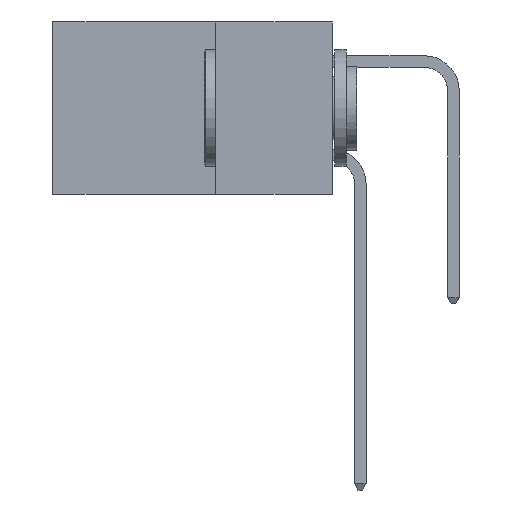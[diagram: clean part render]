
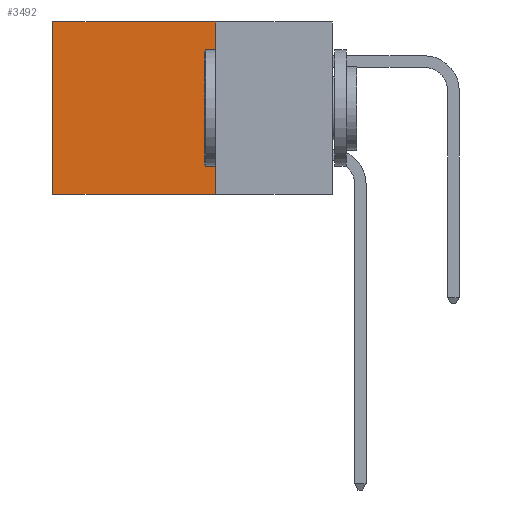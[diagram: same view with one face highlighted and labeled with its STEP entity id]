
A CAD part, left-side view. The second image highlights one B-rep face of the part: STEP entity #3492.
In plain terms, the highlighted planar face has unit normal (-1, 0, 0).
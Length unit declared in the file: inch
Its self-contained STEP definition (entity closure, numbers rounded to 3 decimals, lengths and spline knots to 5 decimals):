
#49 = CARTESIAN_POINT ( 'NONE',  ( 0.2615, 0.6, -0.37 ) ) ;
#805 = LINE ( 'NONE', #8784, #5209 ) ;
#1521 = EDGE_CURVE ( 'NONE', #4899, #5597, #2468, .T. ) ;
#1525 = CARTESIAN_POINT ( 'NONE',  ( 0.2615, 0.25, -0.37 ) ) ;
#1537 = DIRECTION ( 'NONE',  ( 0., 0., -1. ) ) ;
#1586 = DIRECTION ( 'NONE',  ( 1., 0., 0. ) ) ;
#1589 = PLANE ( 'NONE',  #4593 ) ;
#1717 = DIRECTION ( 'NONE',  ( 0., 1., 0. ) ) ;
#1936 = CARTESIAN_POINT ( 'NONE',  ( 0.2615, 0.25, -0.37 ) ) ;
#2258 = CARTESIAN_POINT ( 'NONE',  ( 0.2615, 0.6, -0.37 ) ) ;
#2468 = LINE ( 'NONE', #2258, #6728 ) ;
#3167 = ORIENTED_EDGE ( 'NONE', *, *, #10643, .T. ) ;
#3250 = FACE_OUTER_BOUND ( 'NONE', #10162, .T. ) ;
#3492 = ADVANCED_FACE ( 'NONE', ( #3250 ), #1589, .F. ) ;
#3504 = EDGE_CURVE ( 'NONE', #4692, #5597, #7989, .T. ) ;
#3636 = DIRECTION ( 'NONE',  ( 0., 0., -1. ) ) ;
#3918 = ORIENTED_EDGE ( 'NONE', *, *, #3504, .F. ) ;
#4133 = CARTESIAN_POINT ( 'NONE',  ( 0.2615, 0.6, 0. ) ) ;
#4434 = VERTEX_POINT ( 'NONE', #9902 ) ;
#4531 = ORIENTED_EDGE ( 'NONE', *, *, #9877, .F. ) ;
#4593 = AXIS2_PLACEMENT_3D ( 'NONE', #1936, #1586, #1537 ) ;
#4692 = VERTEX_POINT ( 'NONE', #6961 ) ;
#4899 = VERTEX_POINT ( 'NONE', #4133 ) ;
#4994 = DIRECTION ( 'NONE',  ( 0., 0., -1. ) ) ;
#5209 = VECTOR ( 'NONE', #8028, 39.37008 ) ;
#5597 = VERTEX_POINT ( 'NONE', #49 ) ;
#5765 = VECTOR ( 'NONE', #4994, 39.37008 ) ;
#6027 = LINE ( 'NONE', #9104, #5765 ) ;
#6728 = VECTOR ( 'NONE', #3636, 39.37008 ) ;
#6961 = CARTESIAN_POINT ( 'NONE',  ( 0.2615, 0.25, -0.37 ) ) ;
#7466 = VECTOR ( 'NONE', #1717, 39.37008 ) ;
#7989 = LINE ( 'NONE', #1525, #7466 ) ;
#8028 = DIRECTION ( 'NONE',  ( 0., 1., 0. ) ) ;
#8784 = CARTESIAN_POINT ( 'NONE',  ( 0.2615, 0.25, 0. ) ) ;
#8995 = ORIENTED_EDGE ( 'NONE', *, *, #1521, .T. ) ;
#9104 = CARTESIAN_POINT ( 'NONE',  ( 0.2615, 0.25, -0.37 ) ) ;
#9877 = EDGE_CURVE ( 'NONE', #4434, #4692, #6027, .T. ) ;
#9902 = CARTESIAN_POINT ( 'NONE',  ( 0.2615, 0.25, 0. ) ) ;
#10162 = EDGE_LOOP ( 'NONE', ( #8995, #3918, #4531, #3167 ) ) ;
#10643 = EDGE_CURVE ( 'NONE', #4434, #4899, #805, .T. ) ;
